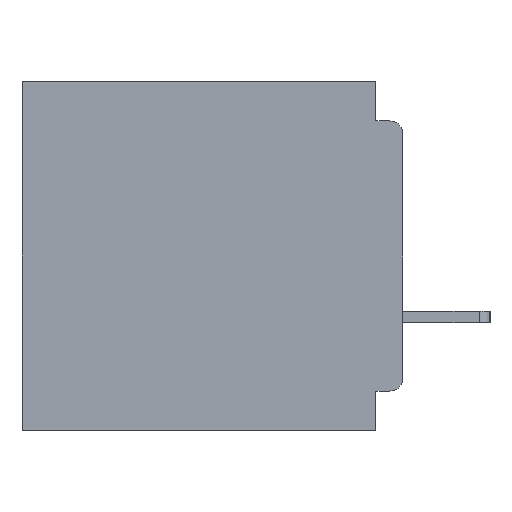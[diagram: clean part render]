
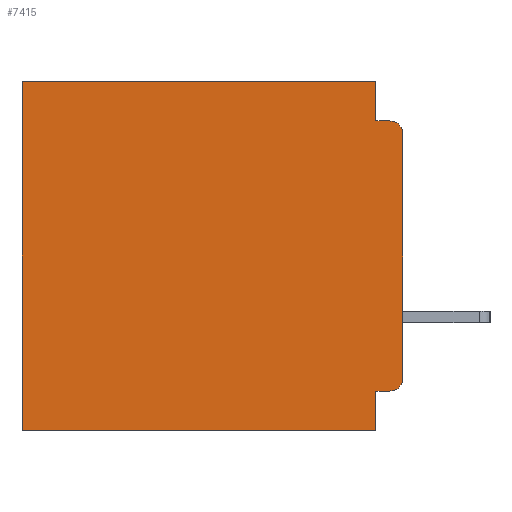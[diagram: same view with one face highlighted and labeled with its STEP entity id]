
A CAD part, left-side view. The second image highlights one B-rep face of the part: STEP entity #7415.
In plain terms, the highlighted planar face has unit normal (-1, 0, 0).
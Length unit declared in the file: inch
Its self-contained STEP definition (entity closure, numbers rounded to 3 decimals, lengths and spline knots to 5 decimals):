
#86 = EDGE_CURVE ( 'NONE', #39549, #31582, #36210, .T. ) ;
#618 = VERTEX_POINT ( 'NONE', #41126 ) ;
#1073 = VECTOR ( 'NONE', #1241, 39.37008 ) ;
#1241 = DIRECTION ( 'NONE',  ( 0., 0., -1. ) ) ;
#1601 = FACE_OUTER_BOUND ( 'NONE', #7372, .T. ) ;
#1796 = ORIENTED_EDGE ( 'NONE', *, *, #9601, .T. ) ;
#2553 = DIRECTION ( 'NONE',  ( 0., 1., 0. ) ) ;
#2639 = VERTEX_POINT ( 'NONE', #11066 ) ;
#2876 = DIRECTION ( 'NONE',  ( 0., 0., -1. ) ) ;
#3126 = VECTOR ( 'NONE', #2553, 39.37008 ) ;
#3658 = CARTESIAN_POINT ( 'NONE',  ( 0.3, 0., -0.4 ) ) ;
#3892 = EDGE_CURVE ( 'NONE', #40271, #13760, #44090, .T. ) ;
#5210 = CARTESIAN_POINT ( 'NONE',  ( 0.3, 0.031, 0. ) ) ;
#5875 = ORIENTED_EDGE ( 'NONE', *, *, #20698, .F. ) ;
#6581 = VERTEX_POINT ( 'NONE', #20901 ) ;
#6912 = CARTESIAN_POINT ( 'NONE',  ( 0.3, 0.031, -0.045 ) ) ;
#7372 = EDGE_LOOP ( 'NONE', ( #38203, #23516, #33747, #5875, #34498, #1796, #26774, #35456, #33593, #41858 ) ) ;
#7415 = ADVANCED_FACE ( 'NONE', ( #1601 ), #14476, .F. ) ;
#7961 = CARTESIAN_POINT ( 'NONE',  ( 0.3, 0., -0.4 ) ) ;
#8330 = VERTEX_POINT ( 'NONE', #5210 ) ;
#9601 = EDGE_CURVE ( 'NONE', #2639, #31582, #40811, .T. ) ;
#10490 = VERTEX_POINT ( 'NONE', #28875 ) ;
#10914 = LINE ( 'NONE', #44828, #1073 ) ;
#11066 = CARTESIAN_POINT ( 'NONE',  ( 0.3, 0.437, 0. ) ) ;
#13076 = CARTESIAN_POINT ( 'NONE',  ( 0.3, 0.031, -0.4 ) ) ;
#13760 = VERTEX_POINT ( 'NONE', #37373 ) ;
#14476 = PLANE ( 'NONE',  #38844 ) ;
#16823 = AXIS2_PLACEMENT_3D ( 'NONE', #21024, #46238, #24727 ) ;
#17067 = EDGE_CURVE ( 'NONE', #39011, #618, #42808, .T. ) ;
#17802 = CARTESIAN_POINT ( 'NONE',  ( 0.3, 0., 0. ) ) ;
#18257 = EDGE_CURVE ( 'NONE', #6581, #39549, #10914, .T. ) ;
#18266 = DIRECTION ( 'NONE',  ( 0., 0., -1. ) ) ;
#19796 = EDGE_CURVE ( 'NONE', #8330, #2639, #45916, .T. ) ;
#20698 = EDGE_CURVE ( 'NONE', #8330, #40271, #25596, .T. ) ;
#20901 = CARTESIAN_POINT ( 'NONE',  ( 0.3, 0.031, -0.355 ) ) ;
#21024 = CARTESIAN_POINT ( 'NONE',  ( 0.3, 0.015, -0.06 ) ) ;
#21348 = CARTESIAN_POINT ( 'NONE',  ( 0.3, 0.015, -0.34 ) ) ;
#21429 = CIRCLE ( 'NONE', #16823, 0.015 ) ;
#21983 = EDGE_CURVE ( 'NONE', #10490, #13760, #21429, .T. ) ;
#23104 = DIRECTION ( 'NONE',  ( 0., 1., 0. ) ) ;
#23516 = ORIENTED_EDGE ( 'NONE', *, *, #21983, .T. ) ;
#23778 = LINE ( 'NONE', #46049, #3126 ) ;
#23796 = VECTOR ( 'NONE', #36781, 39.37008 ) ;
#24727 = DIRECTION ( 'NONE',  ( 0., 0., -1. ) ) ;
#25034 = DIRECTION ( 'NONE',  ( 0., 0., -1. ) ) ;
#25596 = LINE ( 'NONE', #28498, #35303 ) ;
#26774 = ORIENTED_EDGE ( 'NONE', *, *, #86, .F. ) ;
#27398 = AXIS2_PLACEMENT_3D ( 'NONE', #21348, #46528, #25034 ) ;
#28415 = EDGE_CURVE ( 'NONE', #10490, #618, #45677, .T. ) ;
#28498 = CARTESIAN_POINT ( 'NONE',  ( 0.3, 0.031, 0. ) ) ;
#28875 = CARTESIAN_POINT ( 'NONE',  ( 0.3, 0., -0.06 ) ) ;
#29170 = CARTESIAN_POINT ( 'NONE',  ( 0.3, 0., -0.4 ) ) ;
#30844 = DIRECTION ( 'NONE',  ( 0., 0., -1. ) ) ;
#31285 = VECTOR ( 'NONE', #30844, 39.37008 ) ;
#31360 = CARTESIAN_POINT ( 'NONE',  ( 0.3, 0., -0.045 ) ) ;
#31582 = VERTEX_POINT ( 'NONE', #45073 ) ;
#33593 = ORIENTED_EDGE ( 'NONE', *, *, #34211, .F. ) ;
#33747 = ORIENTED_EDGE ( 'NONE', *, *, #3892, .F. ) ;
#34211 = EDGE_CURVE ( 'NONE', #39011, #6581, #23778, .T. ) ;
#34498 = ORIENTED_EDGE ( 'NONE', *, *, #19796, .T. ) ;
#34518 = CARTESIAN_POINT ( 'NONE',  ( 0.3, 0.437, -0.4 ) ) ;
#35139 = VECTOR ( 'NONE', #37190, 39.37008 ) ;
#35303 = VECTOR ( 'NONE', #2876, 39.37008 ) ;
#35456 = ORIENTED_EDGE ( 'NONE', *, *, #18257, .F. ) ;
#35636 = CARTESIAN_POINT ( 'NONE',  ( 0.3, 0.015, -0.355 ) ) ;
#36210 = LINE ( 'NONE', #3658, #44495 ) ;
#36781 = DIRECTION ( 'NONE',  ( 0., -1., 0. ) ) ;
#37190 = DIRECTION ( 'NONE',  ( 0., 0., -1. ) ) ;
#37373 = CARTESIAN_POINT ( 'NONE',  ( 0.3, 0.015, -0.045 ) ) ;
#38203 = ORIENTED_EDGE ( 'NONE', *, *, #28415, .F. ) ;
#38844 = AXIS2_PLACEMENT_3D ( 'NONE', #29170, #40038, #18266 ) ;
#39011 = VERTEX_POINT ( 'NONE', #35636 ) ;
#39549 = VERTEX_POINT ( 'NONE', #13076 ) ;
#40038 = DIRECTION ( 'NONE',  ( 1., 0., 0. ) ) ;
#40271 = VERTEX_POINT ( 'NONE', #6912 ) ;
#40811 = LINE ( 'NONE', #34518, #31285 ) ;
#41126 = CARTESIAN_POINT ( 'NONE',  ( 0.3, 0., -0.34 ) ) ;
#41858 = ORIENTED_EDGE ( 'NONE', *, *, #17067, .T. ) ;
#42808 = CIRCLE ( 'NONE', #27398, 0.015 ) ;
#44090 = LINE ( 'NONE', #31360, #23796 ) ;
#44495 = VECTOR ( 'NONE', #23104, 39.37008 ) ;
#44816 = VECTOR ( 'NONE', #46671, 39.37008 ) ;
#44828 = CARTESIAN_POINT ( 'NONE',  ( 0.3, 0.031, -0.4 ) ) ;
#45073 = CARTESIAN_POINT ( 'NONE',  ( 0.3, 0.437, -0.4 ) ) ;
#45677 = LINE ( 'NONE', #7961, #35139 ) ;
#45916 = LINE ( 'NONE', #17802, #44816 ) ;
#46049 = CARTESIAN_POINT ( 'NONE',  ( 0.3, 0., -0.355 ) ) ;
#46238 = DIRECTION ( 'NONE',  ( -1., 0., 0. ) ) ;
#46528 = DIRECTION ( 'NONE',  ( -1., 0., 0. ) ) ;
#46671 = DIRECTION ( 'NONE',  ( 0., 1., 0. ) ) ;
